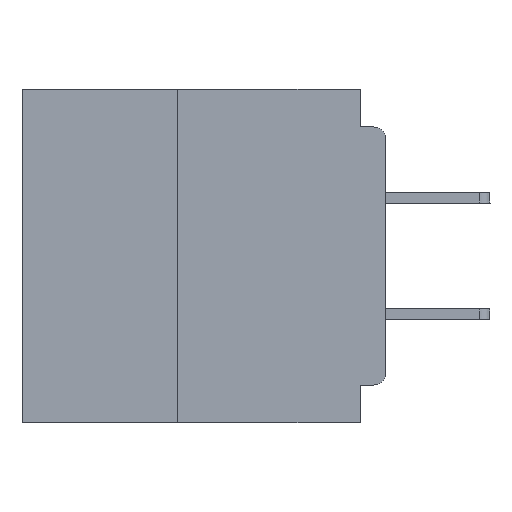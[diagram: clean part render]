
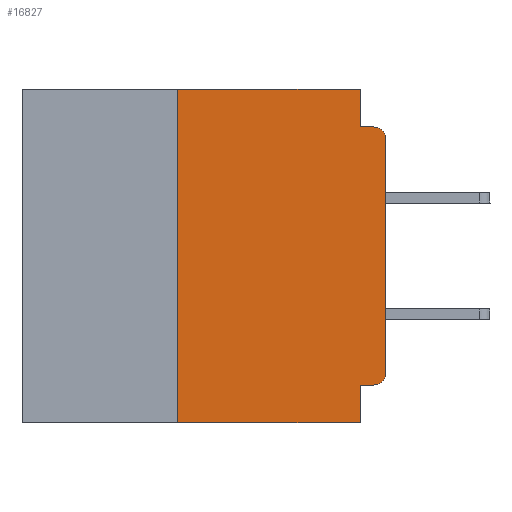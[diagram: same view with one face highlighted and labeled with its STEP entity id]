
A CAD part, left-side view. The second image highlights one B-rep face of the part: STEP entity #16827.
In plain terms, the highlighted planar face has unit normal (-1, 0, 0).
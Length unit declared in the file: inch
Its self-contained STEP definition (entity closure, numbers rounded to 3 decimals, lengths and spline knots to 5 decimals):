
#1477 = DIRECTION ( 'NONE',  ( 1., 0., 0. ) ) ;
#2268 = ORIENTED_EDGE ( 'NONE', *, *, #15996, .F. ) ;
#2289 = VERTEX_POINT ( 'NONE', #36355 ) ;
#3210 = ORIENTED_EDGE ( 'NONE', *, *, #57549, .F. ) ;
#4327 = DIRECTION ( 'NONE',  ( 0., -1., 0. ) ) ;
#5485 = CARTESIAN_POINT ( 'NONE',  ( 0., 0.031, 0. ) ) ;
#5759 = CARTESIAN_POINT ( 'NONE',  ( 0., 0.031, 0. ) ) ;
#6151 = EDGE_CURVE ( 'NONE', #13707, #55036, #9522, .T. ) ;
#6291 = CARTESIAN_POINT ( 'NONE',  ( 0., 0.015, -0.34 ) ) ;
#7005 = ORIENTED_EDGE ( 'NONE', *, *, #56619, .F. ) ;
#7943 = AXIS2_PLACEMENT_3D ( 'NONE', #6291, #42525, #11523 ) ;
#8146 = EDGE_CURVE ( 'NONE', #13655, #66371, #33094, .T. ) ;
#8172 = CARTESIAN_POINT ( 'NONE',  ( 0., 0.25, 0. ) ) ;
#8637 = VERTEX_POINT ( 'NONE', #13425 ) ;
#8653 = DIRECTION ( 'NONE',  ( -1., 0., 0. ) ) ;
#8751 = CARTESIAN_POINT ( 'NONE',  ( 0., 0.031, -0.4 ) ) ;
#9034 = EDGE_CURVE ( 'NONE', #14837, #13655, #17599, .T. ) ;
#9522 = LINE ( 'NONE', #5759, #59609 ) ;
#10045 = AXIS2_PLACEMENT_3D ( 'NONE', #32561, #1477, #37738 ) ;
#11523 = DIRECTION ( 'NONE',  ( 0., 0., -1. ) ) ;
#12262 = EDGE_CURVE ( 'NONE', #55036, #8637, #30242, .T. ) ;
#12289 = CARTESIAN_POINT ( 'NONE',  ( 0., 0.031, -0.4 ) ) ;
#13425 = CARTESIAN_POINT ( 'NONE',  ( 0., 0.015, -0.045 ) ) ;
#13655 = VERTEX_POINT ( 'NONE', #61518 ) ;
#13707 = VERTEX_POINT ( 'NONE', #5485 ) ;
#14837 = VERTEX_POINT ( 'NONE', #35152 ) ;
#15384 = EDGE_LOOP ( 'NONE', ( #46051, #62396, #43428, #18693, #7005, #2268, #60062, #22785, #3210, #64907 ) ) ;
#15996 = EDGE_CURVE ( 'NONE', #2289, #66454, #59663, .T. ) ;
#16447 = VECTOR ( 'NONE', #4327, 39.37008 ) ;
#16827 = ADVANCED_FACE ( 'NONE', ( #33752 ), #22129, .F. ) ;
#17599 = CIRCLE ( 'NONE', #7943, 0.015 ) ;
#18693 = ORIENTED_EDGE ( 'NONE', *, *, #6151, .F. ) ;
#22129 = PLANE ( 'NONE',  #10045 ) ;
#22695 = AXIS2_PLACEMENT_3D ( 'NONE', #39643, #8653, #44808 ) ;
#22785 = ORIENTED_EDGE ( 'NONE', *, *, #40665, .F. ) ;
#25100 = LINE ( 'NONE', #58466, #35565 ) ;
#27899 = VECTOR ( 'NONE', #65655, 39.37008 ) ;
#28342 = CARTESIAN_POINT ( 'NONE',  ( 0., 0., -0.06 ) ) ;
#29513 = LINE ( 'NONE', #8751, #27899 ) ;
#29836 = DIRECTION ( 'NONE',  ( 0., 0., 1. ) ) ;
#30223 = CARTESIAN_POINT ( 'NONE',  ( 0., 0.031, -0.045 ) ) ;
#30242 = LINE ( 'NONE', #66203, #16447 ) ;
#32154 = LINE ( 'NONE', #50770, #57938 ) ;
#32561 = CARTESIAN_POINT ( 'NONE',  ( 0., 0.437, 0. ) ) ;
#32791 = DIRECTION ( 'NONE',  ( 0., -1., 0. ) ) ;
#33094 = LINE ( 'NONE', #44847, #45204 ) ;
#33752 = FACE_OUTER_BOUND ( 'NONE', #15384, .T. ) ;
#35152 = CARTESIAN_POINT ( 'NONE',  ( 0., 0.015, -0.355 ) ) ;
#35565 = VECTOR ( 'NONE', #32791, 39.37008 ) ;
#36355 = CARTESIAN_POINT ( 'NONE',  ( 0., 0.25, -0.4 ) ) ;
#37738 = DIRECTION ( 'NONE',  ( 0., 0., -1. ) ) ;
#37856 = EDGE_CURVE ( 'NONE', #66371, #8637, #65503, .T. ) ;
#39643 = CARTESIAN_POINT ( 'NONE',  ( 0., 0.015, -0.06 ) ) ;
#40053 = CARTESIAN_POINT ( 'NONE',  ( 0., 0.031, -0.355 ) ) ;
#40665 = EDGE_CURVE ( 'NONE', #42834, #51545, #29513, .T. ) ;
#42525 = DIRECTION ( 'NONE',  ( -1., 0., 0. ) ) ;
#42834 = VERTEX_POINT ( 'NONE', #40053 ) ;
#43428 = ORIENTED_EDGE ( 'NONE', *, *, #12262, .F. ) ;
#44808 = DIRECTION ( 'NONE',  ( 0., 0., -1. ) ) ;
#44847 = CARTESIAN_POINT ( 'NONE',  ( 0., 0., 0. ) ) ;
#45204 = VECTOR ( 'NONE', #49790, 39.37008 ) ;
#45979 = VECTOR ( 'NONE', #29836, 39.37008 ) ;
#46051 = ORIENTED_EDGE ( 'NONE', *, *, #8146, .T. ) ;
#49135 = CARTESIAN_POINT ( 'NONE',  ( 0., 0.437, 0. ) ) ;
#49787 = VECTOR ( 'NONE', #64704, 39.37008 ) ;
#49790 = DIRECTION ( 'NONE',  ( 0., 0., 1. ) ) ;
#50770 = CARTESIAN_POINT ( 'NONE',  ( 0., 0., -0.355 ) ) ;
#51545 = VERTEX_POINT ( 'NONE', #12289 ) ;
#52300 = DIRECTION ( 'NONE',  ( 0., 0., -1. ) ) ;
#55036 = VERTEX_POINT ( 'NONE', #30223 ) ;
#56619 = EDGE_CURVE ( 'NONE', #66454, #13707, #63499, .T. ) ;
#57549 = EDGE_CURVE ( 'NONE', #14837, #42834, #32154, .T. ) ;
#57938 = VECTOR ( 'NONE', #61350, 39.37008 ) ;
#58466 = CARTESIAN_POINT ( 'NONE',  ( 0., 0.437, -0.4 ) ) ;
#59609 = VECTOR ( 'NONE', #52300, 39.37008 ) ;
#59663 = LINE ( 'NONE', #60714, #45979 ) ;
#60062 = ORIENTED_EDGE ( 'NONE', *, *, #62235, .T. ) ;
#60714 = CARTESIAN_POINT ( 'NONE',  ( 0., 0.25, -0.4 ) ) ;
#61350 = DIRECTION ( 'NONE',  ( 0., 1., 0. ) ) ;
#61518 = CARTESIAN_POINT ( 'NONE',  ( 0., 0., -0.34 ) ) ;
#62235 = EDGE_CURVE ( 'NONE', #2289, #51545, #25100, .T. ) ;
#62396 = ORIENTED_EDGE ( 'NONE', *, *, #37856, .T. ) ;
#63499 = LINE ( 'NONE', #49135, #49787 ) ;
#64704 = DIRECTION ( 'NONE',  ( 0., -1., 0. ) ) ;
#64907 = ORIENTED_EDGE ( 'NONE', *, *, #9034, .T. ) ;
#65503 = CIRCLE ( 'NONE', #22695, 0.015 ) ;
#65655 = DIRECTION ( 'NONE',  ( 0., 0., -1. ) ) ;
#66203 = CARTESIAN_POINT ( 'NONE',  ( 0., 0., -0.045 ) ) ;
#66371 = VERTEX_POINT ( 'NONE', #28342 ) ;
#66454 = VERTEX_POINT ( 'NONE', #8172 ) ;
